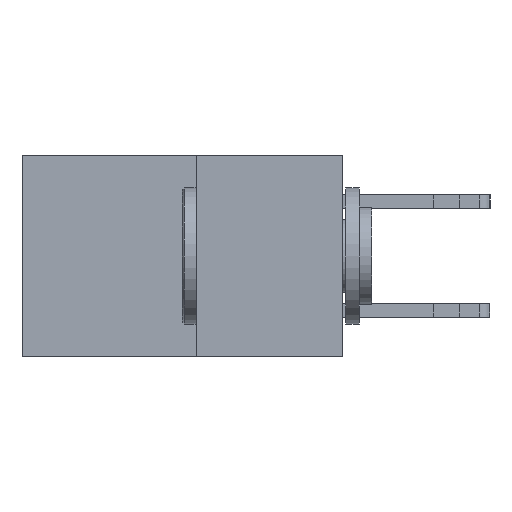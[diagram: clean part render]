
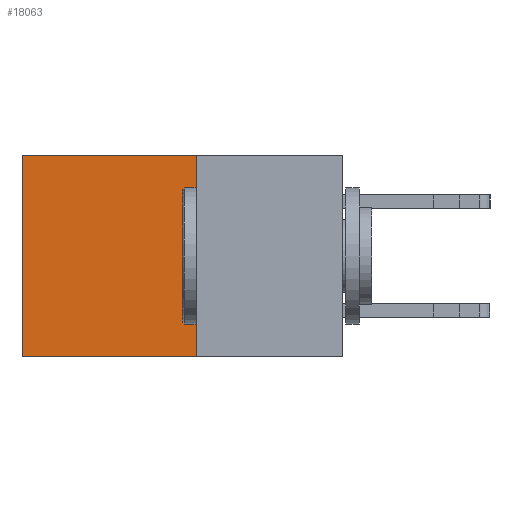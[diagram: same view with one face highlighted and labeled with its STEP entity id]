
A CAD part, left-side view. The second image highlights one B-rep face of the part: STEP entity #18063.
In plain terms, the highlighted planar face has unit normal (-1, 0, 0).
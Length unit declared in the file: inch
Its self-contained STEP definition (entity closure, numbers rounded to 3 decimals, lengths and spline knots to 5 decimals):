
#1322 = LINE ( 'NONE', #8942, #10679 ) ;
#1349 = VERTEX_POINT ( 'NONE', #5511 ) ;
#1563 = VECTOR ( 'NONE', #19855, 39.37008 ) ;
#1990 = EDGE_CURVE ( 'NONE', #22209, #20424, #3686, .T. ) ;
#2437 = VECTOR ( 'NONE', #22187, 39.37008 ) ;
#3003 = EDGE_CURVE ( 'NONE', #19337, #20424, #3640, .T. ) ;
#3640 = LINE ( 'NONE', #20500, #2437 ) ;
#3649 = FACE_OUTER_BOUND ( 'NONE', #17058, .T. ) ;
#3686 = LINE ( 'NONE', #4750, #9200 ) ;
#4750 = CARTESIAN_POINT ( 'NONE',  ( 0.277, 0.27, -0.37 ) ) ;
#5012 = CARTESIAN_POINT ( 'NONE',  ( 0.277, 0.27, -0.37 ) ) ;
#5511 = CARTESIAN_POINT ( 'NONE',  ( 0.277, 0.27, 0. ) ) ;
#6365 = ORIENTED_EDGE ( 'NONE', *, *, #8861, .F. ) ;
#7858 = CARTESIAN_POINT ( 'NONE',  ( 0.277, 0.59, 0. ) ) ;
#8333 = PLANE ( 'NONE',  #20324 ) ;
#8861 = EDGE_CURVE ( 'NONE', #1349, #22209, #1322, .T. ) ;
#8942 = CARTESIAN_POINT ( 'NONE',  ( 0.277, 0.27, -0.37 ) ) ;
#9200 = VECTOR ( 'NONE', #17669, 39.37008 ) ;
#10175 = CARTESIAN_POINT ( 'NONE',  ( 0.277, 0.27, -0.37 ) ) ;
#10679 = VECTOR ( 'NONE', #19961, 39.37008 ) ;
#11037 = CARTESIAN_POINT ( 'NONE',  ( 0.277, 0.59, -0.37 ) ) ;
#11336 = ORIENTED_EDGE ( 'NONE', *, *, #3003, .T. ) ;
#11488 = LINE ( 'NONE', #18012, #1563 ) ;
#12013 = DIRECTION ( 'NONE',  ( 0., 0., -1. ) ) ;
#12405 = ORIENTED_EDGE ( 'NONE', *, *, #1990, .F. ) ;
#14591 = ORIENTED_EDGE ( 'NONE', *, *, #17524, .T. ) ;
#17058 = EDGE_LOOP ( 'NONE', ( #11336, #12405, #6365, #14591 ) ) ;
#17524 = EDGE_CURVE ( 'NONE', #1349, #19337, #11488, .T. ) ;
#17669 = DIRECTION ( 'NONE',  ( 0., 1., 0. ) ) ;
#18012 = CARTESIAN_POINT ( 'NONE',  ( 0.277, 0.27, 0. ) ) ;
#18063 = ADVANCED_FACE ( 'NONE', ( #3649 ), #8333, .F. ) ;
#19337 = VERTEX_POINT ( 'NONE', #7858 ) ;
#19855 = DIRECTION ( 'NONE',  ( 0., 1., 0. ) ) ;
#19961 = DIRECTION ( 'NONE',  ( 0., 0., -1. ) ) ;
#20324 = AXIS2_PLACEMENT_3D ( 'NONE', #10175, #22978, #12013 ) ;
#20424 = VERTEX_POINT ( 'NONE', #11037 ) ;
#20500 = CARTESIAN_POINT ( 'NONE',  ( 0.277, 0.59, -0.37 ) ) ;
#22187 = DIRECTION ( 'NONE',  ( 0., 0., -1. ) ) ;
#22209 = VERTEX_POINT ( 'NONE', #5012 ) ;
#22978 = DIRECTION ( 'NONE',  ( 1., 0., 0. ) ) ;
